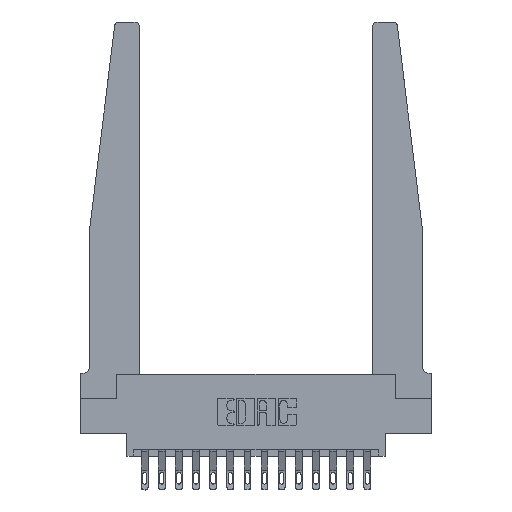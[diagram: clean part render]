
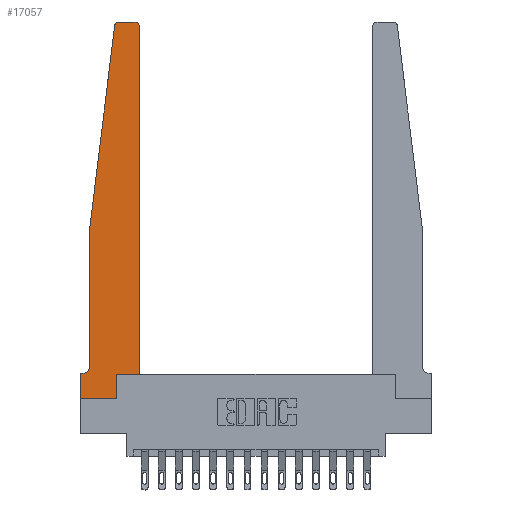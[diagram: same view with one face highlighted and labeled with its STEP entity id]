
A CAD part, top view. The second image highlights one B-rep face of the part: STEP entity #17057.
In plain terms, the highlighted planar face has unit normal (0, 0, 1).
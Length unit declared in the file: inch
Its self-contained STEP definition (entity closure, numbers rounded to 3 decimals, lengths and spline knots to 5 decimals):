
#20 = EDGE_CURVE ( 'NONE', #5509, #10819, #9514, .T. ) ;
#130 = DIRECTION ( 'NONE',  ( 0., -1., 0. ) ) ;
#271 = CARTESIAN_POINT ( 'NONE',  ( 0.425, 0.18, 0.37 ) ) ;
#749 = CARTESIAN_POINT ( 'NONE',  ( 0., 0., 0.37 ) ) ;
#786 = VECTOR ( 'NONE', #130, 39.37008 ) ;
#923 = CARTESIAN_POINT ( 'NONE',  ( 0.015, 0.2375, 0.37 ) ) ;
#1135 = VERTEX_POINT ( 'NONE', #10848 ) ;
#1145 = DIRECTION ( 'NONE',  ( 0., 0., 1. ) ) ;
#1232 = LINE ( 'NONE', #16938, #786 ) ;
#1246 = FACE_OUTER_BOUND ( 'NONE', #9138, .T. ) ;
#1497 = DIRECTION ( 'NONE',  ( 0., 1., 0. ) ) ;
#1524 = VECTOR ( 'NONE', #11911, 39.37008 ) ;
#1745 = CARTESIAN_POINT ( 'NONE',  ( 0.425, 2.72, 0.37 ) ) ;
#1983 = EDGE_CURVE ( 'NONE', #16440, #11548, #5562, .T. ) ;
#2333 = DIRECTION ( 'NONE',  ( -1., 0., 0. ) ) ;
#2511 = CARTESIAN_POINT ( 'NONE',  ( 0.015, 0.1875, 0.37 ) ) ;
#2574 = CARTESIAN_POINT ( 'NONE',  ( 0., 0.1875, 0.37 ) ) ;
#2642 = VECTOR ( 'NONE', #8590, 39.37008 ) ;
#2739 = AXIS2_PLACEMENT_3D ( 'NONE', #923, #10644, #2333 ) ;
#2743 = ORIENTED_EDGE ( 'NONE', *, *, #11777, .T. ) ;
#3099 = CARTESIAN_POINT ( 'NONE',  ( 0.425, 0.18, 0.37 ) ) ;
#3346 = CARTESIAN_POINT ( 'NONE',  ( 0.395, 2.72, 0.37 ) ) ;
#3450 = VECTOR ( 'NONE', #17814, 39.37008 ) ;
#3624 = VECTOR ( 'NONE', #13871, 39.37008 ) ;
#3671 = LINE ( 'NONE', #8593, #9981 ) ;
#3909 = CARTESIAN_POINT ( 'NONE',  ( 0.395, 2.75, 0.37 ) ) ;
#3943 = ORIENTED_EDGE ( 'NONE', *, *, #20, .T. ) ;
#4039 = CIRCLE ( 'NONE', #17563, 0.03 ) ;
#4165 = ORIENTED_EDGE ( 'NONE', *, *, #4632, .T. ) ;
#4226 = CARTESIAN_POINT ( 'NONE',  ( 0.065, 1.25, 0.37 ) ) ;
#4412 = VERTEX_POINT ( 'NONE', #14470 ) ;
#4614 = DIRECTION ( 'NONE',  ( 0., -1., 0. ) ) ;
#4632 = EDGE_CURVE ( 'NONE', #7569, #11568, #13127, .T. ) ;
#4752 = DIRECTION ( 'NONE',  ( 1., 0., 0. ) ) ;
#5117 = EDGE_CURVE ( 'NONE', #4412, #1135, #5233, .T. ) ;
#5204 = ORIENTED_EDGE ( 'NONE', *, *, #6678, .T. ) ;
#5233 = LINE ( 'NONE', #749, #1524 ) ;
#5487 = CARTESIAN_POINT ( 'NONE',  ( 0.065, 1.25, 0.37 ) ) ;
#5509 = VERTEX_POINT ( 'NONE', #3099 ) ;
#5562 = LINE ( 'NONE', #14415, #9683 ) ;
#5645 = DIRECTION ( 'NONE',  ( -1., 0., 0. ) ) ;
#6542 = CARTESIAN_POINT ( 'NONE',  ( 0.25, 2.75, 0.37 ) ) ;
#6678 = EDGE_CURVE ( 'NONE', #10819, #6981, #4039, .T. ) ;
#6757 = DIRECTION ( 'NONE',  ( 0., 0., 1. ) ) ;
#6799 = ORIENTED_EDGE ( 'NONE', *, *, #14868, .T. ) ;
#6981 = VERTEX_POINT ( 'NONE', #3909 ) ;
#7569 = VERTEX_POINT ( 'NONE', #13679 ) ;
#8116 = AXIS2_PLACEMENT_3D ( 'NONE', #2574, #6757, #16622 ) ;
#8370 = VERTEX_POINT ( 'NONE', #11482 ) ;
#8590 = DIRECTION ( 'NONE',  ( 1., 0., 0. ) ) ;
#8593 = CARTESIAN_POINT ( 'NONE',  ( 0.2605, 0.18, 0.37 ) ) ;
#8979 = EDGE_CURVE ( 'NONE', #12936, #14747, #14037, .T. ) ;
#9138 = EDGE_LOOP ( 'NONE', ( #10111, #4165, #14012, #13283, #6799, #17608, #9351, #17648, #2743, #16533, #3943, #5204 ) ) ;
#9351 = ORIENTED_EDGE ( 'NONE', *, *, #17530, .T. ) ;
#9465 = CARTESIAN_POINT ( 'NONE',  ( 0.27653, 2.72, 0.37 ) ) ;
#9495 = PLANE ( 'NONE',  #8116 ) ;
#9514 = LINE ( 'NONE', #9945, #13256 ) ;
#9683 = VECTOR ( 'NONE', #4614, 39.37008 ) ;
#9935 = DIRECTION ( 'NONE',  ( 0., 1., 0. ) ) ;
#9945 = CARTESIAN_POINT ( 'NONE',  ( 0.425, 0.18, 0.37 ) ) ;
#9981 = VECTOR ( 'NONE', #9935, 39.37008 ) ;
#10111 = ORIENTED_EDGE ( 'NONE', *, *, #11594, .T. ) ;
#10644 = DIRECTION ( 'NONE',  ( 0., 0., -1. ) ) ;
#10819 = VERTEX_POINT ( 'NONE', #1745 ) ;
#10848 = CARTESIAN_POINT ( 'NONE',  ( 0.2605, 0., 0.37 ) ) ;
#10867 = DIRECTION ( 'NONE',  ( 1., 0., 0. ) ) ;
#11043 = LINE ( 'NONE', #5487, #3624 ) ;
#11482 = CARTESIAN_POINT ( 'NONE',  ( 0.2605, 0.18, 0.37 ) ) ;
#11548 = VERTEX_POINT ( 'NONE', #13338 ) ;
#11568 = VERTEX_POINT ( 'NONE', #11988 ) ;
#11594 = EDGE_CURVE ( 'NONE', #6981, #7569, #17524, .T. ) ;
#11777 = EDGE_CURVE ( 'NONE', #1135, #8370, #3671, .T. ) ;
#11911 = DIRECTION ( 'NONE',  ( 1., 0., 0. ) ) ;
#11984 = CIRCLE ( 'NONE', #2739, 0.05 ) ;
#11988 = CARTESIAN_POINT ( 'NONE',  ( 0.24675, 2.72367, 0.37 ) ) ;
#12936 = VERTEX_POINT ( 'NONE', #2511 ) ;
#13127 = CIRCLE ( 'NONE', #16602, 0.03 ) ;
#13149 = DIRECTION ( 'NONE',  ( 0., 0., 1. ) ) ;
#13256 = VECTOR ( 'NONE', #1497, 39.37008 ) ;
#13283 = ORIENTED_EDGE ( 'NONE', *, *, #1983, .T. ) ;
#13338 = CARTESIAN_POINT ( 'NONE',  ( 0.065, 0.2375, 0.37 ) ) ;
#13679 = CARTESIAN_POINT ( 'NONE',  ( 0.27653, 2.75, 0.37 ) ) ;
#13770 = EDGE_CURVE ( 'NONE', #8370, #5509, #13795, .T. ) ;
#13795 = LINE ( 'NONE', #271, #2642 ) ;
#13871 = DIRECTION ( 'NONE',  ( -0.122, -0.992, 0. ) ) ;
#14012 = ORIENTED_EDGE ( 'NONE', *, *, #17137, .T. ) ;
#14036 = CARTESIAN_POINT ( 'NONE',  ( 0.065, 0.1875, 0.37 ) ) ;
#14037 = LINE ( 'NONE', #14036, #17807 ) ;
#14415 = CARTESIAN_POINT ( 'NONE',  ( 0.065, 1.25, 0.37 ) ) ;
#14470 = CARTESIAN_POINT ( 'NONE',  ( 0., 0., 0.37 ) ) ;
#14747 = VERTEX_POINT ( 'NONE', #17420 ) ;
#14868 = EDGE_CURVE ( 'NONE', #11548, #12936, #11984, .T. ) ;
#16440 = VERTEX_POINT ( 'NONE', #4226 ) ;
#16533 = ORIENTED_EDGE ( 'NONE', *, *, #13770, .T. ) ;
#16602 = AXIS2_PLACEMENT_3D ( 'NONE', #9465, #1145, #10867 ) ;
#16622 = DIRECTION ( 'NONE',  ( 1., 0., 0. ) ) ;
#16938 = CARTESIAN_POINT ( 'NONE',  ( 0., 0., 0.37 ) ) ;
#17057 = ADVANCED_FACE ( 'NONE', ( #1246 ), #9495, .T. ) ;
#17137 = EDGE_CURVE ( 'NONE', #11568, #16440, #11043, .T. ) ;
#17420 = CARTESIAN_POINT ( 'NONE',  ( 0., 0.1875, 0.37 ) ) ;
#17524 = LINE ( 'NONE', #6542, #3450 ) ;
#17530 = EDGE_CURVE ( 'NONE', #14747, #4412, #1232, .T. ) ;
#17563 = AXIS2_PLACEMENT_3D ( 'NONE', #3346, #13149, #4752 ) ;
#17608 = ORIENTED_EDGE ( 'NONE', *, *, #8979, .T. ) ;
#17648 = ORIENTED_EDGE ( 'NONE', *, *, #5117, .T. ) ;
#17807 = VECTOR ( 'NONE', #5645, 39.37008 ) ;
#17814 = DIRECTION ( 'NONE',  ( -1., 0., 0. ) ) ;
